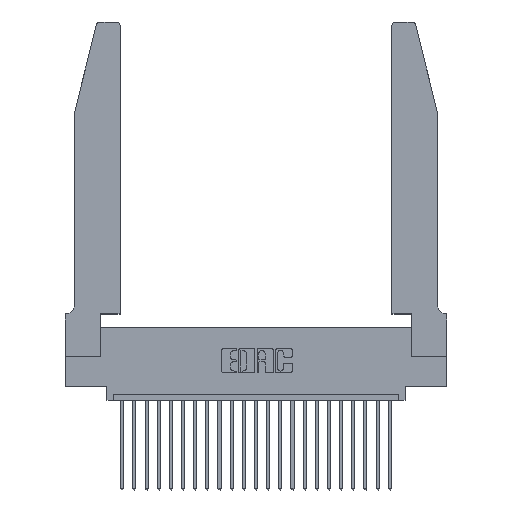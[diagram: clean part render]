
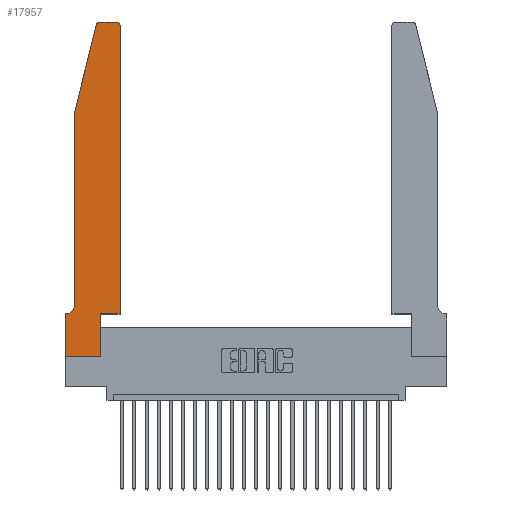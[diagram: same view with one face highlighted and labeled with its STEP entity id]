
A CAD part, top view. The second image highlights one B-rep face of the part: STEP entity #17957.
In plain terms, the highlighted planar face has unit normal (0, 0, 1).
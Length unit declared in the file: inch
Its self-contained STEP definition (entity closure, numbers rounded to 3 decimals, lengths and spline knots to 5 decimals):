
#239 = ORIENTED_EDGE ( 'NONE', *, *, #8514, .T. ) ;
#419 = CIRCLE ( 'NONE', #13019, 0.03 ) ;
#553 = VERTEX_POINT ( 'NONE', #10728 ) ;
#778 = DIRECTION ( 'NONE',  ( 0., 0., 1. ) ) ;
#810 = CARTESIAN_POINT ( 'NONE',  ( 0.0755, 2., 0.37 ) ) ;
#1226 = LINE ( 'NONE', #14308, #3567 ) ;
#1361 = LINE ( 'NONE', #810, #16046 ) ;
#1402 = VECTOR ( 'NONE', #19222, 39.37008 ) ;
#1923 = VECTOR ( 'NONE', #18524, 39.37008 ) ;
#2141 = VERTEX_POINT ( 'NONE', #16423 ) ;
#2155 = VERTEX_POINT ( 'NONE', #10867 ) ;
#2608 = VERTEX_POINT ( 'NONE', #13742 ) ;
#3265 = VERTEX_POINT ( 'NONE', #12324 ) ;
#3283 = VERTEX_POINT ( 'NONE', #21926 ) ;
#3567 = VECTOR ( 'NONE', #4416, 39.37008 ) ;
#3654 = DIRECTION ( 'NONE',  ( 0., 0., -1. ) ) ;
#3888 = ORIENTED_EDGE ( 'NONE', *, *, #15395, .T. ) ;
#4416 = DIRECTION ( 'NONE',  ( 1., 0., 0. ) ) ;
#4469 = EDGE_LOOP ( 'NONE', ( #239, #17050, #5012, #16058, #23561, #12965, #3888, #5215, #6303, #11563, #13683, #16150 ) ) ;
#5012 = ORIENTED_EDGE ( 'NONE', *, *, #20075, .T. ) ;
#5057 = CARTESIAN_POINT ( 'NONE',  ( 0.284, 2.72, 0.37 ) ) ;
#5215 = ORIENTED_EDGE ( 'NONE', *, *, #17191, .T. ) ;
#5773 = VERTEX_POINT ( 'NONE', #7132 ) ;
#6206 = AXIS2_PLACEMENT_3D ( 'NONE', #5057, #7154, #18466 ) ;
#6248 = CARTESIAN_POINT ( 'NONE',  ( 0.2605, 2.75, 0.37 ) ) ;
#6293 = CARTESIAN_POINT ( 'NONE',  ( 0.25487, 2.72718, 0.37 ) ) ;
#6303 = ORIENTED_EDGE ( 'NONE', *, *, #17363, .T. ) ;
#6574 = VERTEX_POINT ( 'NONE', #6293 ) ;
#6627 = CARTESIAN_POINT ( 'NONE',  ( 0.4505, 0.35, 0.37 ) ) ;
#6658 = DIRECTION ( 'NONE',  ( 0., -1., 0. ) ) ;
#6737 = CARTESIAN_POINT ( 'NONE',  ( 0.4205, 2.75, 0.37 ) ) ;
#6930 = DIRECTION ( 'NONE',  ( 1., 0., 0. ) ) ;
#7132 = CARTESIAN_POINT ( 'NONE',  ( 0.0755, 0.42, 0.37 ) ) ;
#7154 = DIRECTION ( 'NONE',  ( 0., 0., 1. ) ) ;
#7598 = EDGE_CURVE ( 'NONE', #553, #16574, #419, .T. ) ;
#8006 = VERTEX_POINT ( 'NONE', #23639 ) ;
#8416 = VERTEX_POINT ( 'NONE', #6627 ) ;
#8450 = EDGE_CURVE ( 'NONE', #5773, #2141, #15612, .T. ) ;
#8514 = EDGE_CURVE ( 'NONE', #16574, #2608, #8780, .T. ) ;
#8780 = LINE ( 'NONE', #6248, #13512 ) ;
#9586 = VECTOR ( 'NONE', #14223, 39.37008 ) ;
#9782 = LINE ( 'NONE', #10300, #21402 ) ;
#9871 = CIRCLE ( 'NONE', #6206, 0.03 ) ;
#10216 = DIRECTION ( 'NONE',  ( -1., 0., 0. ) ) ;
#10270 = CARTESIAN_POINT ( 'NONE',  ( 0., 0., 0.37 ) ) ;
#10300 = CARTESIAN_POINT ( 'NONE',  ( 0.0755, 0.35, 0.37 ) ) ;
#10336 = EDGE_CURVE ( 'NONE', #2141, #3283, #9782, .T. ) ;
#10696 = DIRECTION ( 'NONE',  ( 0., 1., 0. ) ) ;
#10728 = CARTESIAN_POINT ( 'NONE',  ( 0.4505, 2.72, 0.37 ) ) ;
#10744 = LINE ( 'NONE', #19147, #1402 ) ;
#10867 = CARTESIAN_POINT ( 'NONE',  ( 0.2865, 0., 0.37 ) ) ;
#11019 = CARTESIAN_POINT ( 'NONE',  ( 0.2865, 0.35, 0.37 ) ) ;
#11090 = CARTESIAN_POINT ( 'NONE',  ( 0., 0., 0.37 ) ) ;
#11563 = ORIENTED_EDGE ( 'NONE', *, *, #12844, .T. ) ;
#12261 = CARTESIAN_POINT ( 'NONE',  ( 0.4205, 2.72, 0.37 ) ) ;
#12324 = CARTESIAN_POINT ( 'NONE',  ( 0.2865, 0.35, 0.37 ) ) ;
#12718 = PLANE ( 'NONE',  #15894 ) ;
#12800 = DIRECTION ( 'NONE',  ( 0., 0., 1. ) ) ;
#12844 = EDGE_CURVE ( 'NONE', #3265, #8416, #1226, .T. ) ;
#12855 = VECTOR ( 'NONE', #10696, 39.37008 ) ;
#12965 = ORIENTED_EDGE ( 'NONE', *, *, #10336, .T. ) ;
#13019 = AXIS2_PLACEMENT_3D ( 'NONE', #12261, #778, #24115 ) ;
#13512 = VECTOR ( 'NONE', #14337, 39.37008 ) ;
#13683 = ORIENTED_EDGE ( 'NONE', *, *, #23847, .T. ) ;
#13742 = CARTESIAN_POINT ( 'NONE',  ( 0.284, 2.75, 0.37 ) ) ;
#14223 = DIRECTION ( 'NONE',  ( 1., 0., 0. ) ) ;
#14308 = CARTESIAN_POINT ( 'NONE',  ( 0.4505, 0.35, 0.37 ) ) ;
#14337 = DIRECTION ( 'NONE',  ( -1., 0., 0. ) ) ;
#15131 = LINE ( 'NONE', #11090, #21153 ) ;
#15217 = LINE ( 'NONE', #10270, #9586 ) ;
#15337 = VERTEX_POINT ( 'NONE', #24673 ) ;
#15395 = EDGE_CURVE ( 'NONE', #3283, #15337, #15131, .T. ) ;
#15612 = CIRCLE ( 'NONE', #17035, 0.07 ) ;
#15894 = AXIS2_PLACEMENT_3D ( 'NONE', #18411, #12800, #6930 ) ;
#15985 = EDGE_CURVE ( 'NONE', #8006, #5773, #1361, .T. ) ;
#16046 = VECTOR ( 'NONE', #6658, 39.37008 ) ;
#16058 = ORIENTED_EDGE ( 'NONE', *, *, #15985, .T. ) ;
#16150 = ORIENTED_EDGE ( 'NONE', *, *, #7598, .T. ) ;
#16423 = CARTESIAN_POINT ( 'NONE',  ( 0.0055, 0.35, 0.37 ) ) ;
#16574 = VERTEX_POINT ( 'NONE', #6737 ) ;
#16670 = CARTESIAN_POINT ( 'NONE',  ( 0.0755, 2., 0.37 ) ) ;
#16735 = LINE ( 'NONE', #11019, #12855 ) ;
#17035 = AXIS2_PLACEMENT_3D ( 'NONE', #17246, #3654, #17332 ) ;
#17050 = ORIENTED_EDGE ( 'NONE', *, *, #22955, .T. ) ;
#17191 = EDGE_CURVE ( 'NONE', #15337, #2155, #15217, .T. ) ;
#17246 = CARTESIAN_POINT ( 'NONE',  ( 0.0055, 0.42, 0.37 ) ) ;
#17332 = DIRECTION ( 'NONE',  ( -1., 0., 0. ) ) ;
#17363 = EDGE_CURVE ( 'NONE', #2155, #3265, #16735, .T. ) ;
#17957 = ADVANCED_FACE ( 'NONE', ( #23272 ), #12718, .T. ) ;
#18411 = CARTESIAN_POINT ( 'NONE',  ( 0., 0.35, 0.37 ) ) ;
#18466 = DIRECTION ( 'NONE',  ( 1., 0., 0. ) ) ;
#18524 = DIRECTION ( 'NONE',  ( -0.239, -0.971, 0. ) ) ;
#19147 = CARTESIAN_POINT ( 'NONE',  ( 0.4505, 0.35, 0.37 ) ) ;
#19222 = DIRECTION ( 'NONE',  ( 0., 1., 0. ) ) ;
#20075 = EDGE_CURVE ( 'NONE', #6574, #8006, #22883, .T. ) ;
#21153 = VECTOR ( 'NONE', #22891, 39.37008 ) ;
#21402 = VECTOR ( 'NONE', #10216, 39.37008 ) ;
#21926 = CARTESIAN_POINT ( 'NONE',  ( 0., 0.35, 0.37 ) ) ;
#22883 = LINE ( 'NONE', #16670, #1923 ) ;
#22891 = DIRECTION ( 'NONE',  ( 0., -1., 0. ) ) ;
#22955 = EDGE_CURVE ( 'NONE', #2608, #6574, #9871, .T. ) ;
#23272 = FACE_OUTER_BOUND ( 'NONE', #4469, .T. ) ;
#23561 = ORIENTED_EDGE ( 'NONE', *, *, #8450, .T. ) ;
#23639 = CARTESIAN_POINT ( 'NONE',  ( 0.0755, 2., 0.37 ) ) ;
#23847 = EDGE_CURVE ( 'NONE', #8416, #553, #10744, .T. ) ;
#24115 = DIRECTION ( 'NONE',  ( 1., 0., 0. ) ) ;
#24673 = CARTESIAN_POINT ( 'NONE',  ( 0., 0., 0.37 ) ) ;
